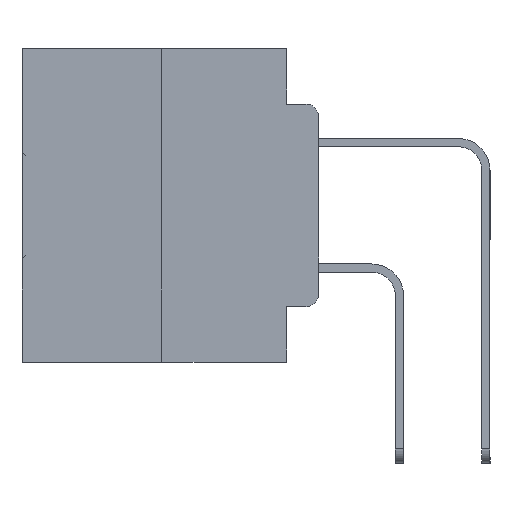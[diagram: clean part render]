
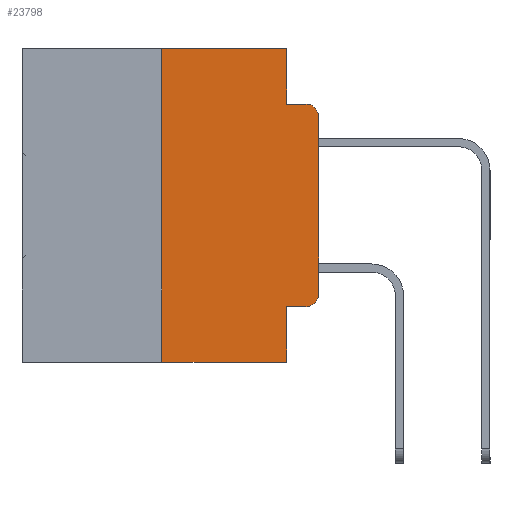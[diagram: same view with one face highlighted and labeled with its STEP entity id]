
A CAD part, left-side view. The second image highlights one B-rep face of the part: STEP entity #23798.
In plain terms, the highlighted planar face has unit normal (-1, 0, 0).
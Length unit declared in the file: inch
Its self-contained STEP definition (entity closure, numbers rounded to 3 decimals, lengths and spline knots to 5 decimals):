
#961 = ORIENTED_EDGE ( 'NONE', *, *, #13609, .T. ) ;
#1208 = ORIENTED_EDGE ( 'NONE', *, *, #8428, .T. ) ;
#1214 = EDGE_CURVE ( 'NONE', #22443, #18757, #9523, .T. ) ;
#1345 = ORIENTED_EDGE ( 'NONE', *, *, #1214, .F. ) ;
#1470 = VECTOR ( 'NONE', #7907, 39.37008 ) ;
#1622 = CARTESIAN_POINT ( 'NONE',  ( 0., 0., 0. ) ) ;
#1685 = CARTESIAN_POINT ( 'NONE',  ( 0., 0.473, 0. ) ) ;
#2321 = CARTESIAN_POINT ( 'NONE',  ( 0., 0.051, -0.0885 ) ) ;
#2825 = ORIENTED_EDGE ( 'NONE', *, *, #23221, .T. ) ;
#3908 = VERTEX_POINT ( 'NONE', #7698 ) ;
#3926 = CARTESIAN_POINT ( 'NONE',  ( 0., 0.051, -0.4115 ) ) ;
#4178 = VERTEX_POINT ( 'NONE', #18851 ) ;
#4713 = LINE ( 'NONE', #31492, #24251 ) ;
#4892 = ORIENTED_EDGE ( 'NONE', *, *, #5535, .F. ) ;
#4912 = DIRECTION ( 'NONE',  ( -1., 0., 0. ) ) ;
#5218 = CARTESIAN_POINT ( 'NONE',  ( 0., 0.25, 0. ) ) ;
#5535 = EDGE_CURVE ( 'NONE', #24639, #4178, #15986, .T. ) ;
#5669 = ORIENTED_EDGE ( 'NONE', *, *, #20973, .F. ) ;
#6639 = ORIENTED_EDGE ( 'NONE', *, *, #20198, .F. ) ;
#6844 = ORIENTED_EDGE ( 'NONE', *, *, #27595, .F. ) ;
#7029 = LINE ( 'NONE', #1685, #14706 ) ;
#7159 = VERTEX_POINT ( 'NONE', #12228 ) ;
#7599 = CARTESIAN_POINT ( 'NONE',  ( 0., 0., -0.3915 ) ) ;
#7652 = CARTESIAN_POINT ( 'NONE',  ( 0., 0.473, 0. ) ) ;
#7698 = CARTESIAN_POINT ( 'NONE',  ( 0., 0.25, -0.5 ) ) ;
#7907 = DIRECTION ( 'NONE',  ( 0., 0., 1. ) ) ;
#7947 = VECTOR ( 'NONE', #29338, 39.37008 ) ;
#8428 = EDGE_CURVE ( 'NONE', #23073, #18757, #22603, .T. ) ;
#8449 = VERTEX_POINT ( 'NONE', #7599 ) ;
#8967 = CARTESIAN_POINT ( 'NONE',  ( 0., 0.051, -0.0885 ) ) ;
#8983 = DIRECTION ( 'NONE',  ( 0., 0., -1. ) ) ;
#9209 = ORIENTED_EDGE ( 'NONE', *, *, #24521, .T. ) ;
#9523 = LINE ( 'NONE', #2321, #22906 ) ;
#9618 = AXIS2_PLACEMENT_3D ( 'NONE', #27154, #12210, #29653 ) ;
#9657 = DIRECTION ( 'NONE',  ( 0., -1., 0. ) ) ;
#10302 = DIRECTION ( 'NONE',  ( 0., 0., -1. ) ) ;
#10616 = AXIS2_PLACEMENT_3D ( 'NONE', #20286, #4912, #22764 ) ;
#11380 = CARTESIAN_POINT ( 'NONE',  ( 0., 0.051, -0.4115 ) ) ;
#11445 = CARTESIAN_POINT ( 'NONE',  ( 0., 0.02, -0.0885 ) ) ;
#12210 = DIRECTION ( 'NONE',  ( -1., 0., 0. ) ) ;
#12228 = CARTESIAN_POINT ( 'NONE',  ( 0., 0.051, 0. ) ) ;
#13609 = EDGE_CURVE ( 'NONE', #8449, #23073, #23615, .T. ) ;
#14054 = DIRECTION ( 'NONE',  ( 0., 0., -1. ) ) ;
#14706 = VECTOR ( 'NONE', #9657, 39.37008 ) ;
#14738 = DIRECTION ( 'NONE',  ( 0., 0., 1. ) ) ;
#14785 = LINE ( 'NONE', #3926, #7947 ) ;
#15175 = AXIS2_PLACEMENT_3D ( 'NONE', #7652, #25313, #10302 ) ;
#15207 = VECTOR ( 'NONE', #8983, 39.37008 ) ;
#15469 = CARTESIAN_POINT ( 'NONE',  ( 0., 0.02, -0.4115 ) ) ;
#15986 = LINE ( 'NONE', #29143, #15207 ) ;
#16058 = DIRECTION ( 'NONE',  ( 0., -1., 0. ) ) ;
#16201 = VECTOR ( 'NONE', #14738, 39.37008 ) ;
#17727 = CARTESIAN_POINT ( 'NONE',  ( 0., 0.25, 0. ) ) ;
#18366 = ORIENTED_EDGE ( 'NONE', *, *, #29888, .T. ) ;
#18757 = VERTEX_POINT ( 'NONE', #11445 ) ;
#18851 = CARTESIAN_POINT ( 'NONE',  ( 0., 0.051, -0.5 ) ) ;
#20198 = EDGE_CURVE ( 'NONE', #32573, #7159, #7029, .T. ) ;
#20286 = CARTESIAN_POINT ( 'NONE',  ( 0., 0.02, -0.1085 ) ) ;
#20336 = PLANE ( 'NONE',  #15175 ) ;
#20973 = EDGE_CURVE ( 'NONE', #3908, #32573, #28639, .T. ) ;
#21066 = CARTESIAN_POINT ( 'NONE',  ( 0., 0.473, -0.5 ) ) ;
#22443 = VERTEX_POINT ( 'NONE', #8967 ) ;
#22603 = CIRCLE ( 'NONE', #10616, 0.02 ) ;
#22764 = DIRECTION ( 'NONE',  ( 0., 0., -1. ) ) ;
#22906 = VECTOR ( 'NONE', #16058, 39.37008 ) ;
#23073 = VERTEX_POINT ( 'NONE', #28892 ) ;
#23221 = EDGE_CURVE ( 'NONE', #31279, #8449, #25045, .T. ) ;
#23535 = DIRECTION ( 'NONE',  ( 0., -1., 0. ) ) ;
#23615 = LINE ( 'NONE', #1622, #16201 ) ;
#23798 = ADVANCED_FACE ( 'NONE', ( #26962 ), #20336, .F. ) ;
#24251 = VECTOR ( 'NONE', #14054, 39.37008 ) ;
#24479 = VECTOR ( 'NONE', #23535, 39.37008 ) ;
#24521 = EDGE_CURVE ( 'NONE', #3908, #4178, #31873, .T. ) ;
#24639 = VERTEX_POINT ( 'NONE', #11380 ) ;
#25045 = CIRCLE ( 'NONE', #9618, 0.02 ) ;
#25313 = DIRECTION ( 'NONE',  ( 1., 0., 0. ) ) ;
#26006 = EDGE_LOOP ( 'NONE', ( #961, #1208, #1345, #6844, #6639, #5669, #9209, #4892, #18366, #2825 ) ) ;
#26962 = FACE_OUTER_BOUND ( 'NONE', #26006, .T. ) ;
#27154 = CARTESIAN_POINT ( 'NONE',  ( 0., 0.02, -0.3915 ) ) ;
#27595 = EDGE_CURVE ( 'NONE', #7159, #22443, #4713, .T. ) ;
#28639 = LINE ( 'NONE', #5218, #1470 ) ;
#28892 = CARTESIAN_POINT ( 'NONE',  ( 0., 0., -0.1085 ) ) ;
#29143 = CARTESIAN_POINT ( 'NONE',  ( 0., 0.051, 0. ) ) ;
#29338 = DIRECTION ( 'NONE',  ( 0., -1., 0. ) ) ;
#29653 = DIRECTION ( 'NONE',  ( 0., 0., -1. ) ) ;
#29888 = EDGE_CURVE ( 'NONE', #24639, #31279, #14785, .T. ) ;
#31279 = VERTEX_POINT ( 'NONE', #15469 ) ;
#31492 = CARTESIAN_POINT ( 'NONE',  ( 0., 0.051, 0. ) ) ;
#31873 = LINE ( 'NONE', #21066, #24479 ) ;
#32573 = VERTEX_POINT ( 'NONE', #17727 ) ;
